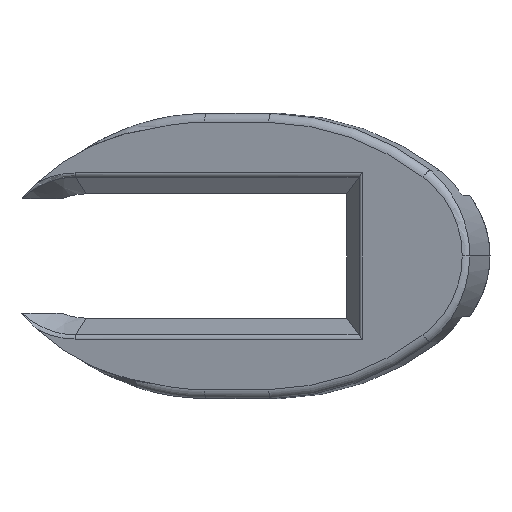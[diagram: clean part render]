
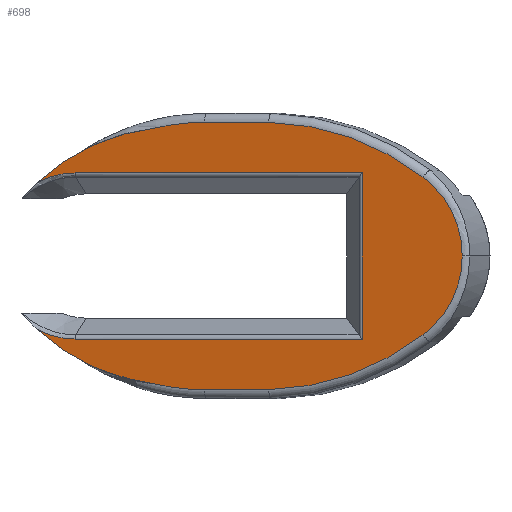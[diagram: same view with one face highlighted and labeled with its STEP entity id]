
A CAD part, front view. The second image highlights one B-rep face of the part: STEP entity #698.
In plain terms, the highlighted planar face has unit normal (-0.25, -0.968, 0).
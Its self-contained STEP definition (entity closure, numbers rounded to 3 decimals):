
#20 = ORIENTED_EDGE ( 'NONE', *, *, #2166, .T. ) ;
#47 = ORIENTED_EDGE ( 'NONE', *, *, #2065, .T. ) ;
#58 = EDGE_CURVE ( 'NONE', #169, #64, #1336, .T. ) ;
#64 = VERTEX_POINT ( 'NONE', #1047 ) ;
#72 = ORIENTED_EDGE ( 'NONE', *, *, #2300, .T. ) ;
#82 = EDGE_CURVE ( 'NONE', #827, #169, #384, .T. ) ;
#103 = AXIS2_PLACEMENT_3D ( 'NONE', #714, #695, #687 ) ;
#105 = CARTESIAN_POINT ( 'NONE',  ( -35.601, 0.464, 9.311 ) ) ;
#106 = AXIS2_PLACEMENT_3D ( 'NONE', #1429, #1419, #1411 ) ;
#125 = EDGE_CURVE ( 'NONE', #426, #1986, #1306, .T. ) ;
#140 = CARTESIAN_POINT ( 'NONE',  ( -39.832, 1.558, -8.272 ) ) ;
#153 = CARTESIAN_POINT ( 'NONE',  ( -13.838, -5.164, -15.027 ) ) ;
#158 = DIRECTION ( 'NONE',  ( -0.968, 0.25, 0. ) ) ;
#161 = CARTESIAN_POINT ( 'NONE',  ( -23.833, -2.579, -10.307 ) ) ;
#167 = AXIS2_PLACEMENT_3D ( 'NONE', #536, #525, #480 ) ;
#169 = VERTEX_POINT ( 'NONE', #140 ) ;
#171 = CARTESIAN_POINT ( 'NONE',  ( -26.452, -1.902, 14.391 ) ) ;
#173 = CARTESIAN_POINT ( 'NONE',  ( -13.838, -5.164, 15.002 ) ) ;
#199 = DIRECTION ( 'NONE',  ( -0.968, 0.25, 0. ) ) ;
#209 = CARTESIAN_POINT ( 'NONE',  ( -21.042, -3.301, -15.027 ) ) ;
#232 = DIRECTION ( 'NONE',  ( -0.25, -0.968, 0. ) ) ;
#316 = VERTEX_POINT ( 'NONE', #809 ) ;
#330 = ORIENTED_EDGE ( 'NONE', *, *, #82, .T. ) ;
#337 = CARTESIAN_POINT ( 'NONE',  ( -3.333, -7.881, -8.998 ) ) ;
#350 = DIRECTION ( 'NONE',  ( 0.968, -0.25, 0. ) ) ;
#384 = CIRCLE ( 'NONE', #103, 9.508 ) ;
#392 = DIRECTION ( 'NONE',  ( -0.968, 0.25, 0. ) ) ;
#423 = CIRCLE ( 'NONE', #1717, 24.846 ) ;
#426 = VERTEX_POINT ( 'NONE', #1060 ) ;
#445 = EDGE_CURVE ( 'NONE', #64, #2181, #1430, .T. ) ;
#480 = DIRECTION ( 'NONE',  ( -0.968, 0.25, 0. ) ) ;
#525 = DIRECTION ( 'NONE',  ( 0.25, 0.968, 0. ) ) ;
#530 = CARTESIAN_POINT ( 'NONE',  ( -2.664, -8.054, -0.025 ) ) ;
#536 = CARTESIAN_POINT ( 'NONE',  ( -35.601, 0.464, -0.197 ) ) ;
#553 = CARTESIAN_POINT ( 'NONE',  ( -3.333, -7.881, 9.311 ) ) ;
#598 = LINE ( 'NONE', #337, #1507 ) ;
#604 = EDGE_CURVE ( 'NONE', #2181, #1012, #659, .T. ) ;
#612 = VECTOR ( 'NONE', #1005, 1000. ) ;
#643 = CIRCLE ( 'NONE', #1568, 31.075 ) ;
#659 = LINE ( 'NONE', #992, #612 ) ;
#687 = DIRECTION ( 'NONE',  ( -0.968, 0.25, 0. ) ) ;
#695 = DIRECTION ( 'NONE',  ( 0.25, 0.968, 0. ) ) ;
#698 = ADVANCED_FACE ( 'NONE', ( #1873 ), #1938, .F. ) ;
#705 = DIRECTION ( 'NONE',  ( -0.968, 0.25, 0. ) ) ;
#714 = CARTESIAN_POINT ( 'NONE',  ( -35.601, 0.464, 0.172 ) ) ;
#734 = EDGE_CURVE ( 'NONE', #2077, #426, #423, .T. ) ;
#765 = DIRECTION ( 'NONE',  ( -0.25, -0.968, 0. ) ) ;
#809 = CARTESIAN_POINT ( 'NONE',  ( 3.48, -9.643, 8.825 ) ) ;
#827 = VERTEX_POINT ( 'NONE', #2086 ) ;
#832 = CIRCLE ( 'NONE', #1185, 31.075 ) ;
#864 = DIRECTION ( 'NONE',  ( 0.25, 0.968, 0. ) ) ;
#872 = VECTOR ( 'NONE', #1837, 1000. ) ;
#890 = AXIS2_PLACEMENT_3D ( 'NONE', #1746, #1589, #1420 ) ;
#945 = LINE ( 'NONE', #2170, #1842 ) ;
#968 = EDGE_CURVE ( 'NONE', #2202, #2077, #1994, .T. ) ;
#992 = CARTESIAN_POINT ( 'NONE',  ( -14.534, -4.984, -15.027 ) ) ;
#1005 = DIRECTION ( 'NONE',  ( 0.968, -0.25, 0. ) ) ;
#1012 = VERTEX_POINT ( 'NONE', #153 ) ;
#1047 = CARTESIAN_POINT ( 'NONE',  ( -26.452, -1.902, -14.417 ) ) ;
#1054 = VERTEX_POINT ( 'NONE', #553 ) ;
#1060 = CARTESIAN_POINT ( 'NONE',  ( -39.832, 1.558, 8.247 ) ) ;
#1075 = CARTESIAN_POINT ( 'NONE',  ( -21.042, -3.301, -10.872 ) ) ;
#1133 = CIRCLE ( 'NONE', #1333, 10.89 ) ;
#1185 = AXIS2_PLACEMENT_3D ( 'NONE', #2338, #1269, #158 ) ;
#1198 = EDGE_CURVE ( 'NONE', #1012, #2352, #643, .T. ) ;
#1253 = DIRECTION ( 'NONE',  ( -0.968, 0.25, 0. ) ) ;
#1259 = DIRECTION ( 'NONE',  ( 0., 0., -1. ) ) ;
#1269 = DIRECTION ( 'NONE',  ( -0.25, -0.968, 0. ) ) ;
#1306 = CIRCLE ( 'NONE', #167, 9.508 ) ;
#1322 = CARTESIAN_POINT ( 'NONE',  ( 3.48, -9.643, -8.85 ) ) ;
#1333 = AXIS2_PLACEMENT_3D ( 'NONE', #530, #1781, #705 ) ;
#1335 = CARTESIAN_POINT ( 'NONE',  ( -2.664, -8.054, 0. ) ) ;
#1336 = CIRCLE ( 'NONE', #106, 24.846 ) ;
#1411 = DIRECTION ( 'NONE',  ( -0.968, 0.25, 0. ) ) ;
#1419 = DIRECTION ( 'NONE',  ( -0.25, -0.968, 0. ) ) ;
#1420 = DIRECTION ( 'NONE',  ( -0.968, 0.25, 0. ) ) ;
#1424 = AXIS2_PLACEMENT_3D ( 'NONE', #1335, #232, #1522 ) ;
#1429 = CARTESIAN_POINT ( 'NONE',  ( -23.833, -2.579, 10.282 ) ) ;
#1430 = CIRCLE ( 'NONE', #890, 25.874 ) ;
#1460 = DIRECTION ( 'NONE',  ( -0.25, -0.968, 0. ) ) ;
#1495 = CARTESIAN_POINT ( 'NONE',  ( -35.601, 0.464, -9.336 ) ) ;
#1507 = VECTOR ( 'NONE', #1259, 1000. ) ;
#1522 = DIRECTION ( 'NONE',  ( -0.968, 0.25, 0. ) ) ;
#1568 = AXIS2_PLACEMENT_3D ( 'NONE', #1845, #765, #2028 ) ;
#1587 = VERTEX_POINT ( 'NONE', #2168 ) ;
#1589 = DIRECTION ( 'NONE',  ( -0.25, -0.968, 0. ) ) ;
#1606 = AXIS2_PLACEMENT_3D ( 'NONE', #1075, #2328, #1253 ) ;
#1648 = VECTOR ( 'NONE', #392, 1000. ) ;
#1661 = CARTESIAN_POINT ( 'NONE',  ( -3.616, -7.808, 9.311 ) ) ;
#1690 = ORIENTED_EDGE ( 'NONE', *, *, #58, .T. ) ;
#1714 = VERTEX_POINT ( 'NONE', #1820 ) ;
#1717 = AXIS2_PLACEMENT_3D ( 'NONE', #161, #1460, #350 ) ;
#1722 = AXIS2_PLACEMENT_3D ( 'NONE', #1949, #864, #2131 ) ;
#1723 = VERTEX_POINT ( 'NONE', #173 ) ;
#1746 = CARTESIAN_POINT ( 'NONE',  ( -21.042, -3.301, 10.846 ) ) ;
#1781 = DIRECTION ( 'NONE',  ( -0.25, -0.968, 0. ) ) ;
#1787 = ORIENTED_EDGE ( 'NONE', *, *, #445, .T. ) ;
#1820 = CARTESIAN_POINT ( 'NONE',  ( 7.879, -10.78, -0.012 ) ) ;
#1837 = DIRECTION ( 'NONE',  ( 0.968, -0.25, 0. ) ) ;
#1842 = VECTOR ( 'NONE', #199, 1000. ) ;
#1845 = CARTESIAN_POINT ( 'NONE',  ( -14.534, -4.984, 16.039 ) ) ;
#1860 = ORIENTED_EDGE ( 'NONE', *, *, #604, .T. ) ;
#1873 = FACE_OUTER_BOUND ( 'NONE', #1930, .T. ) ;
#1908 = ORIENTED_EDGE ( 'NONE', *, *, #1198, .T. ) ;
#1915 = EDGE_CURVE ( 'NONE', #2352, #1714, #2303, .T. ) ;
#1930 = EDGE_LOOP ( 'NONE', ( #1690, #1787, #1860, #1908, #1934, #1997, #2108, #2161, #2221, #2331, #2362, #20, #47, #72, #330 ) ) ;
#1934 = ORIENTED_EDGE ( 'NONE', *, *, #1915, .T. ) ;
#1938 = PLANE ( 'NONE',  #1722 ) ;
#1949 = CARTESIAN_POINT ( 'NONE',  ( -14.534, -4.984, 16.039 ) ) ;
#1986 = VERTEX_POINT ( 'NONE', #105 ) ;
#1994 = CIRCLE ( 'NONE', #1606, 25.874 ) ;
#1997 = ORIENTED_EDGE ( 'NONE', *, *, #2054, .T. ) ;
#2028 = DIRECTION ( 'NONE',  ( -0.968, 0.25, 0. ) ) ;
#2030 = CARTESIAN_POINT ( 'NONE',  ( -21.042, -3.301, 15.002 ) ) ;
#2054 = EDGE_CURVE ( 'NONE', #1714, #316, #1133, .T. ) ;
#2065 = EDGE_CURVE ( 'NONE', #1054, #1587, #598, .T. ) ;
#2077 = VERTEX_POINT ( 'NONE', #171 ) ;
#2086 = CARTESIAN_POINT ( 'NONE',  ( -35.601, 0.464, -9.336 ) ) ;
#2108 = ORIENTED_EDGE ( 'NONE', *, *, #2109, .T. ) ;
#2109 = EDGE_CURVE ( 'NONE', #316, #1723, #832, .T. ) ;
#2117 = LINE ( 'NONE', #1495, #1648 ) ;
#2131 = DIRECTION ( 'NONE',  ( -0.968, 0.25, 0. ) ) ;
#2161 = ORIENTED_EDGE ( 'NONE', *, *, #2163, .T. ) ;
#2163 = EDGE_CURVE ( 'NONE', #1723, #2202, #945, .T. ) ;
#2166 = EDGE_CURVE ( 'NONE', #1986, #1054, #2314, .T. ) ;
#2168 = CARTESIAN_POINT ( 'NONE',  ( -3.333, -7.881, -9.336 ) ) ;
#2170 = CARTESIAN_POINT ( 'NONE',  ( -14.534, -4.984, 15.002 ) ) ;
#2181 = VERTEX_POINT ( 'NONE', #209 ) ;
#2202 = VERTEX_POINT ( 'NONE', #2030 ) ;
#2221 = ORIENTED_EDGE ( 'NONE', *, *, #968, .T. ) ;
#2300 = EDGE_CURVE ( 'NONE', #1587, #827, #2117, .T. ) ;
#2303 = CIRCLE ( 'NONE', #1424, 10.89 ) ;
#2314 = LINE ( 'NONE', #1661, #872 ) ;
#2328 = DIRECTION ( 'NONE',  ( -0.25, -0.968, 0. ) ) ;
#2331 = ORIENTED_EDGE ( 'NONE', *, *, #734, .T. ) ;
#2338 = CARTESIAN_POINT ( 'NONE',  ( -14.534, -4.984, -16.064 ) ) ;
#2352 = VERTEX_POINT ( 'NONE', #1322 ) ;
#2362 = ORIENTED_EDGE ( 'NONE', *, *, #125, .T. ) ;
